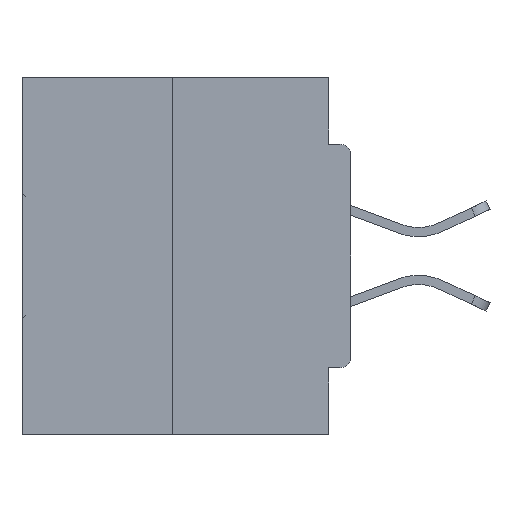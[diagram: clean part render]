
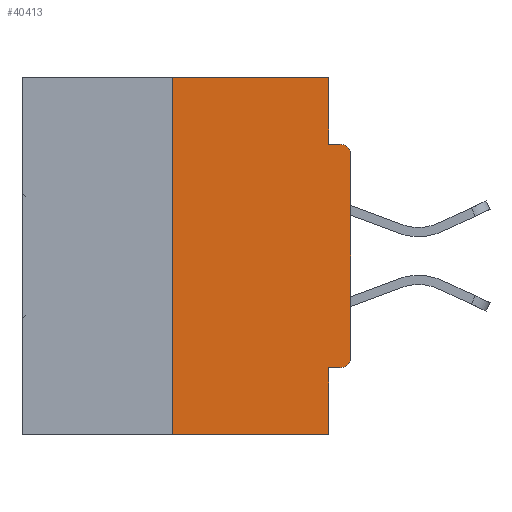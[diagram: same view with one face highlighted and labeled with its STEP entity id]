
A CAD part, left-side view. The second image highlights one B-rep face of the part: STEP entity #40413.
In plain terms, the highlighted planar face has unit normal (-1, 0, 0).
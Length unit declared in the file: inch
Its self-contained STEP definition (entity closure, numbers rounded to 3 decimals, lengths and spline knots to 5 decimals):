
#424 = CIRCLE ( 'NONE', #31870, 0.015 ) ;
#1222 = LINE ( 'NONE', #11516, #40441 ) ;
#1540 = VECTOR ( 'NONE', #16797, 39.37008 ) ;
#2130 = ORIENTED_EDGE ( 'NONE', *, *, #35167, .T. ) ;
#2323 = EDGE_CURVE ( 'NONE', #30610, #22638, #18329, .T. ) ;
#2340 = CARTESIAN_POINT ( 'NONE',  ( 0., 0., -0.1085 ) ) ;
#4246 = DIRECTION ( 'NONE',  ( 0., 0., 1. ) ) ;
#4619 = CARTESIAN_POINT ( 'NONE',  ( 0., 0.015, -0.3915 ) ) ;
#5049 = CARTESIAN_POINT ( 'NONE',  ( 0., 0., -0.3915 ) ) ;
#5379 = DIRECTION ( 'NONE',  ( 1., 0., 0. ) ) ;
#5449 = DIRECTION ( 'NONE',  ( 0., 0., -1. ) ) ;
#8369 = AXIS2_PLACEMENT_3D ( 'NONE', #36481, #5379, #18810 ) ;
#8697 = VECTOR ( 'NONE', #37720, 39.37008 ) ;
#10720 = DIRECTION ( 'NONE',  ( 0., -1., 0. ) ) ;
#11057 = VERTEX_POINT ( 'NONE', #34370 ) ;
#11348 = DIRECTION ( 'NONE',  ( -1., 0., 0. ) ) ;
#11516 = CARTESIAN_POINT ( 'NONE',  ( 0., 0.031, 0. ) ) ;
#11573 = VECTOR ( 'NONE', #10720, 39.37008 ) ;
#11729 = ORIENTED_EDGE ( 'NONE', *, *, #30578, .T. ) ;
#11937 = ORIENTED_EDGE ( 'NONE', *, *, #38932, .F. ) ;
#11958 = CARTESIAN_POINT ( 'NONE',  ( 0., 0.015, -0.4065 ) ) ;
#12151 = EDGE_CURVE ( 'NONE', #11057, #17656, #34624, .T. ) ;
#12329 = PLANE ( 'NONE',  #8369 ) ;
#12555 = VECTOR ( 'NONE', #4246, 39.37008 ) ;
#13224 = CARTESIAN_POINT ( 'NONE',  ( 0., 0.46, -0.5 ) ) ;
#14466 = ORIENTED_EDGE ( 'NONE', *, *, #2323, .F. ) ;
#15644 = CARTESIAN_POINT ( 'NONE',  ( 0., 0., -0.0935 ) ) ;
#15708 = CARTESIAN_POINT ( 'NONE',  ( 0., 0.031, -0.5 ) ) ;
#16728 = EDGE_LOOP ( 'NONE', ( #22057, #23360, #2130, #41579, #11937, #11729, #22333, #19225, #14466, #24840 ) ) ;
#16797 = DIRECTION ( 'NONE',  ( 0., -1., 0. ) ) ;
#17656 = VERTEX_POINT ( 'NONE', #43857 ) ;
#17903 = EDGE_CURVE ( 'NONE', #17656, #23404, #27723, .T. ) ;
#18329 = LINE ( 'NONE', #15644, #39992 ) ;
#18810 = DIRECTION ( 'NONE',  ( 0., 0., -1. ) ) ;
#19225 = ORIENTED_EDGE ( 'NONE', *, *, #26523, .T. ) ;
#20904 = VERTEX_POINT ( 'NONE', #15708 ) ;
#22057 = ORIENTED_EDGE ( 'NONE', *, *, #17903, .F. ) ;
#22333 = ORIENTED_EDGE ( 'NONE', *, *, #39063, .T. ) ;
#22638 = VERTEX_POINT ( 'NONE', #33621 ) ;
#23360 = ORIENTED_EDGE ( 'NONE', *, *, #12151, .F. ) ;
#23404 = VERTEX_POINT ( 'NONE', #31975 ) ;
#23493 = LINE ( 'NONE', #13224, #1540 ) ;
#23871 = CARTESIAN_POINT ( 'NONE',  ( 0., 0.25, 0. ) ) ;
#23921 = CARTESIAN_POINT ( 'NONE',  ( 0., 0.031, -0.4065 ) ) ;
#24178 = DIRECTION ( 'NONE',  ( 0., 1., 0. ) ) ;
#24840 = ORIENTED_EDGE ( 'NONE', *, *, #31082, .F. ) ;
#25150 = DIRECTION ( 'NONE',  ( -1., 0., 0. ) ) ;
#26523 = EDGE_CURVE ( 'NONE', #29829, #22638, #43433, .T. ) ;
#26901 = EDGE_CURVE ( 'NONE', #39230, #20904, #36682, .T. ) ;
#27723 = LINE ( 'NONE', #41355, #11573 ) ;
#29072 = DIRECTION ( 'NONE',  ( 0., 0., -1. ) ) ;
#29307 = VERTEX_POINT ( 'NONE', #11958 ) ;
#29829 = VERTEX_POINT ( 'NONE', #2340 ) ;
#30433 = VECTOR ( 'NONE', #24178, 39.37008 ) ;
#30576 = AXIS2_PLACEMENT_3D ( 'NONE', #36114, #25150, #5449 ) ;
#30578 = EDGE_CURVE ( 'NONE', #29307, #43736, #424, .T. ) ;
#30610 = VERTEX_POINT ( 'NONE', #31500 ) ;
#30934 = CARTESIAN_POINT ( 'NONE',  ( 0., 0., -0.4065 ) ) ;
#31082 = EDGE_CURVE ( 'NONE', #23404, #30610, #1222, .T. ) ;
#31500 = CARTESIAN_POINT ( 'NONE',  ( 0., 0.031, -0.0935 ) ) ;
#31870 = AXIS2_PLACEMENT_3D ( 'NONE', #4619, #11348, #35724 ) ;
#31975 = CARTESIAN_POINT ( 'NONE',  ( 0., 0.031, 0. ) ) ;
#33621 = CARTESIAN_POINT ( 'NONE',  ( 0., 0.015, -0.0935 ) ) ;
#34370 = CARTESIAN_POINT ( 'NONE',  ( 0., 0.25, -0.5 ) ) ;
#34624 = LINE ( 'NONE', #23871, #8697 ) ;
#34912 = LINE ( 'NONE', #41838, #12555 ) ;
#35151 = DIRECTION ( 'NONE',  ( 0., -1., 0. ) ) ;
#35167 = EDGE_CURVE ( 'NONE', #11057, #20904, #23493, .T. ) ;
#35724 = DIRECTION ( 'NONE',  ( 0., 0., -1. ) ) ;
#36114 = CARTESIAN_POINT ( 'NONE',  ( 0., 0.015, -0.1085 ) ) ;
#36481 = CARTESIAN_POINT ( 'NONE',  ( 0., 0.46, 0. ) ) ;
#36682 = LINE ( 'NONE', #43603, #39166 ) ;
#37720 = DIRECTION ( 'NONE',  ( 0., 0., 1. ) ) ;
#37819 = LINE ( 'NONE', #30934, #30433 ) ;
#38932 = EDGE_CURVE ( 'NONE', #29307, #39230, #37819, .T. ) ;
#39020 = DIRECTION ( 'NONE',  ( 0., 0., -1. ) ) ;
#39063 = EDGE_CURVE ( 'NONE', #43736, #29829, #34912, .T. ) ;
#39166 = VECTOR ( 'NONE', #29072, 39.37008 ) ;
#39230 = VERTEX_POINT ( 'NONE', #23921 ) ;
#39828 = FACE_OUTER_BOUND ( 'NONE', #16728, .T. ) ;
#39992 = VECTOR ( 'NONE', #35151, 39.37008 ) ;
#40413 = ADVANCED_FACE ( 'NONE', ( #39828 ), #12329, .F. ) ;
#40441 = VECTOR ( 'NONE', #39020, 39.37008 ) ;
#41355 = CARTESIAN_POINT ( 'NONE',  ( 0., 0.46, 0. ) ) ;
#41579 = ORIENTED_EDGE ( 'NONE', *, *, #26901, .F. ) ;
#41838 = CARTESIAN_POINT ( 'NONE',  ( 0., 0., 0. ) ) ;
#43433 = CIRCLE ( 'NONE', #30576, 0.015 ) ;
#43603 = CARTESIAN_POINT ( 'NONE',  ( 0., 0.031, -0.5 ) ) ;
#43736 = VERTEX_POINT ( 'NONE', #5049 ) ;
#43857 = CARTESIAN_POINT ( 'NONE',  ( 0., 0.25, 0. ) ) ;
